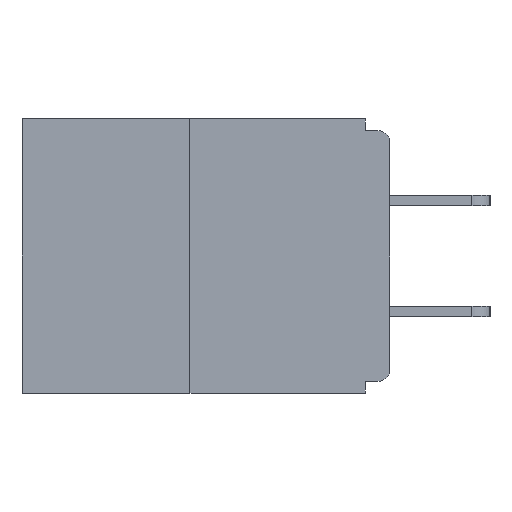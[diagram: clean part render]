
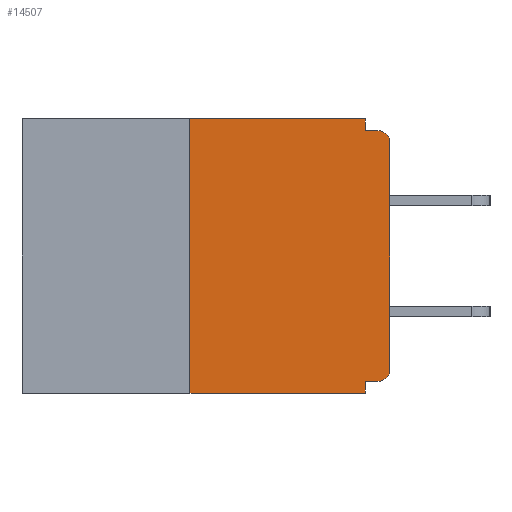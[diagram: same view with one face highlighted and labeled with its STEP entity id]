
A CAD part, left-side view. The second image highlights one B-rep face of the part: STEP entity #14507.
In plain terms, the highlighted planar face has unit normal (-1, 0, 0).
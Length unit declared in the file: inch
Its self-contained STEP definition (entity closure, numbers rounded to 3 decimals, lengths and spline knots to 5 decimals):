
#429 = CARTESIAN_POINT ( 'NONE',  ( 0., 0., -0.313 ) ) ;
#938 = CARTESIAN_POINT ( 'NONE',  ( 0., 0., -0.015 ) ) ;
#985 = CARTESIAN_POINT ( 'NONE',  ( 0., 0.015, -0.328 ) ) ;
#1429 = VECTOR ( 'NONE', #18619, 39.37008 ) ;
#2003 = CARTESIAN_POINT ( 'NONE',  ( 0., 0.031, 0. ) ) ;
#2106 = CARTESIAN_POINT ( 'NONE',  ( 0., 0., 0. ) ) ;
#2203 = VECTOR ( 'NONE', #15009, 39.37008 ) ;
#2432 = ORIENTED_EDGE ( 'NONE', *, *, #2776, .F. ) ;
#2776 = EDGE_CURVE ( 'NONE', #9878, #13738, #16398, .T. ) ;
#3124 = VERTEX_POINT ( 'NONE', #429 ) ;
#3756 = LINE ( 'NONE', #2106, #17194 ) ;
#3937 = CIRCLE ( 'NONE', #6777, 0.015 ) ;
#4197 = EDGE_CURVE ( 'NONE', #20549, #8296, #8012, .T. ) ;
#4653 = DIRECTION ( 'NONE',  ( 0., 0., -1. ) ) ;
#4944 = EDGE_CURVE ( 'NONE', #3124, #7773, #3756, .T. ) ;
#4949 = DIRECTION ( 'NONE',  ( 0., 0., -1. ) ) ;
#5176 = CARTESIAN_POINT ( 'NONE',  ( 0., 0.031, -0.343 ) ) ;
#5462 = CARTESIAN_POINT ( 'NONE',  ( 0., 0.015, -0.313 ) ) ;
#5492 = EDGE_CURVE ( 'NONE', #19992, #6113, #13580, .T. ) ;
#6030 = CARTESIAN_POINT ( 'NONE',  ( 0., 0.46, 0. ) ) ;
#6113 = VERTEX_POINT ( 'NONE', #12752 ) ;
#6139 = ORIENTED_EDGE ( 'NONE', *, *, #4944, .T. ) ;
#6388 = EDGE_CURVE ( 'NONE', #8573, #20549, #8852, .T. ) ;
#6482 = EDGE_LOOP ( 'NONE', ( #9549, #2432, #9838, #14774, #15551, #10163, #6139, #7099, #9220, #8127 ) ) ;
#6777 = AXIS2_PLACEMENT_3D ( 'NONE', #18174, #19811, #4949 ) ;
#7007 = EDGE_CURVE ( 'NONE', #9409, #19992, #21308, .T. ) ;
#7039 = CARTESIAN_POINT ( 'NONE',  ( 0., 0.031, -0.015 ) ) ;
#7099 = ORIENTED_EDGE ( 'NONE', *, *, #15573, .T. ) ;
#7310 = CARTESIAN_POINT ( 'NONE',  ( 0., 0., -0.03 ) ) ;
#7773 = VERTEX_POINT ( 'NONE', #7310 ) ;
#7911 = DIRECTION ( 'NONE',  ( 0., 1., 0. ) ) ;
#8012 = LINE ( 'NONE', #938, #21580 ) ;
#8127 = ORIENTED_EDGE ( 'NONE', *, *, #6388, .F. ) ;
#8296 = VERTEX_POINT ( 'NONE', #11259 ) ;
#8508 = LINE ( 'NONE', #13808, #19822 ) ;
#8573 = VERTEX_POINT ( 'NONE', #14612 ) ;
#8594 = VECTOR ( 'NONE', #15298, 39.37008 ) ;
#8852 = LINE ( 'NONE', #2003, #1429 ) ;
#9220 = ORIENTED_EDGE ( 'NONE', *, *, #4197, .F. ) ;
#9409 = VERTEX_POINT ( 'NONE', #985 ) ;
#9549 = ORIENTED_EDGE ( 'NONE', *, *, #17057, .F. ) ;
#9704 = AXIS2_PLACEMENT_3D ( 'NONE', #5462, #12216, #4653 ) ;
#9838 = ORIENTED_EDGE ( 'NONE', *, *, #11252, .T. ) ;
#9878 = VERTEX_POINT ( 'NONE', #16076 ) ;
#10007 = CARTESIAN_POINT ( 'NONE',  ( 0., 0.46, 0. ) ) ;
#10163 = ORIENTED_EDGE ( 'NONE', *, *, #19925, .T. ) ;
#10227 = LINE ( 'NONE', #10007, #8594 ) ;
#10610 = PLANE ( 'NONE',  #11839 ) ;
#10725 = DIRECTION ( 'NONE',  ( 1., 0., 0. ) ) ;
#11103 = DIRECTION ( 'NONE',  ( 0., -1., 0. ) ) ;
#11252 = EDGE_CURVE ( 'NONE', #9878, #6113, #8508, .T. ) ;
#11259 = CARTESIAN_POINT ( 'NONE',  ( 0., 0.015, -0.015 ) ) ;
#11349 = DIRECTION ( 'NONE',  ( 0., 0., 1. ) ) ;
#11839 = AXIS2_PLACEMENT_3D ( 'NONE', #6030, #10725, #15780 ) ;
#11870 = VECTOR ( 'NONE', #11349, 39.37008 ) ;
#12216 = DIRECTION ( 'NONE',  ( -1., 0., 0. ) ) ;
#12372 = FACE_OUTER_BOUND ( 'NONE', #6482, .T. ) ;
#12752 = CARTESIAN_POINT ( 'NONE',  ( 0., 0.031, -0.343 ) ) ;
#12977 = CARTESIAN_POINT ( 'NONE',  ( 0., 0.031, -0.328 ) ) ;
#13580 = LINE ( 'NONE', #5176, #2203 ) ;
#13738 = VERTEX_POINT ( 'NONE', #15056 ) ;
#13808 = CARTESIAN_POINT ( 'NONE',  ( 0., 0.46, -0.343 ) ) ;
#14299 = VECTOR ( 'NONE', #7911, 39.37008 ) ;
#14507 = ADVANCED_FACE ( 'NONE', ( #12372 ), #10610, .F. ) ;
#14612 = CARTESIAN_POINT ( 'NONE',  ( 0., 0.031, 0. ) ) ;
#14774 = ORIENTED_EDGE ( 'NONE', *, *, #5492, .F. ) ;
#15009 = DIRECTION ( 'NONE',  ( 0., 0., -1. ) ) ;
#15056 = CARTESIAN_POINT ( 'NONE',  ( 0., 0.25, 0. ) ) ;
#15298 = DIRECTION ( 'NONE',  ( 0., -1., 0. ) ) ;
#15551 = ORIENTED_EDGE ( 'NONE', *, *, #7007, .F. ) ;
#15553 = DIRECTION ( 'NONE',  ( 0., -1., 0. ) ) ;
#15573 = EDGE_CURVE ( 'NONE', #7773, #8296, #3937, .T. ) ;
#15780 = DIRECTION ( 'NONE',  ( 0., 0., -1. ) ) ;
#16076 = CARTESIAN_POINT ( 'NONE',  ( 0., 0.25, -0.343 ) ) ;
#16261 = CARTESIAN_POINT ( 'NONE',  ( 0., 0., -0.328 ) ) ;
#16398 = LINE ( 'NONE', #18030, #11870 ) ;
#17057 = EDGE_CURVE ( 'NONE', #13738, #8573, #10227, .T. ) ;
#17194 = VECTOR ( 'NONE', #17209, 39.37008 ) ;
#17209 = DIRECTION ( 'NONE',  ( 0., 0., 1. ) ) ;
#18030 = CARTESIAN_POINT ( 'NONE',  ( 0., 0.25, 0. ) ) ;
#18174 = CARTESIAN_POINT ( 'NONE',  ( 0., 0.015, -0.03 ) ) ;
#18619 = DIRECTION ( 'NONE',  ( 0., 0., -1. ) ) ;
#19153 = CIRCLE ( 'NONE', #9704, 0.015 ) ;
#19811 = DIRECTION ( 'NONE',  ( -1., 0., 0. ) ) ;
#19822 = VECTOR ( 'NONE', #15553, 39.37008 ) ;
#19925 = EDGE_CURVE ( 'NONE', #9409, #3124, #19153, .T. ) ;
#19992 = VERTEX_POINT ( 'NONE', #12977 ) ;
#20549 = VERTEX_POINT ( 'NONE', #7039 ) ;
#21308 = LINE ( 'NONE', #16261, #14299 ) ;
#21580 = VECTOR ( 'NONE', #11103, 39.37008 ) ;
